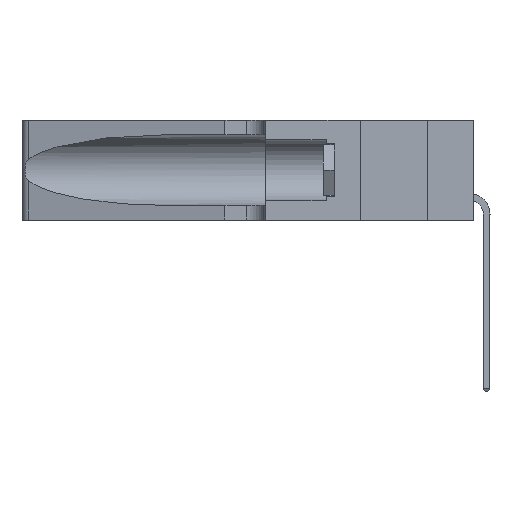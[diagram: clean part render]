
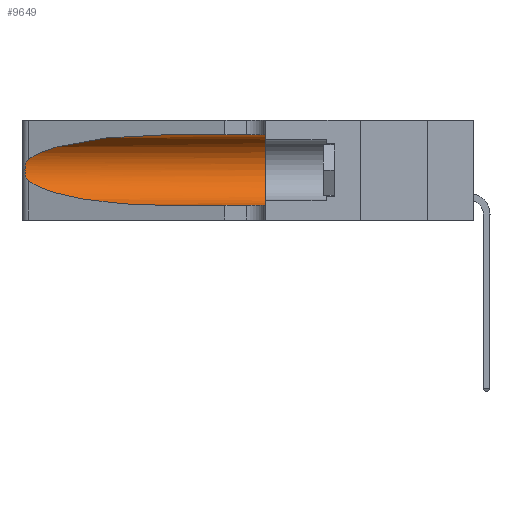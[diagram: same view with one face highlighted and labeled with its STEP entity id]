
A CAD part, left-side view. The second image highlights one B-rep face of the part: STEP entity #9649.
In plain terms, the highlighted cylindrical face has radius 3.308 mm (diameter 6.617 mm), a partial arc.
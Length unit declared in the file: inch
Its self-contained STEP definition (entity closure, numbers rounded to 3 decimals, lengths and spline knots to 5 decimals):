
#487 = CARTESIAN_POINT ( 'NONE',  ( 0.25789, 1.23486, 0.15765 ) ) ;
#1350 = VECTOR ( 'NONE', #30710, 39.37008 ) ;
#1384 = CARTESIAN_POINT ( 'NONE',  ( 0.2373, 1.15595, 0.28018 ) ) ;
#1556 = CARTESIAN_POINT ( 'NONE',  ( 0.1305, 0.72297, 0.31525 ) ) ;
#2177 = ORIENTED_EDGE ( 'NONE', *, *, #15404, .T. ) ;
#2580 = LINE ( 'NONE', #40165, #47400 ) ;
#2984 = ORIENTED_EDGE ( 'NONE', *, *, #41375, .T. ) ;
#3879 = VERTEX_POINT ( 'NONE', #7950 ) ;
#4218 = ORIENTED_EDGE ( 'NONE', *, *, #9594, .F. ) ;
#4560 = CARTESIAN_POINT ( 'NONE',  ( 0.25639, 1.23184, 0.21858 ) ) ;
#5374 =( BOUNDED_CURVE ( )  B_SPLINE_CURVE ( 3, ( #1556, #9085, #1384, #12860 ),
 .UNSPECIFIED., .F., .T. ) 
 B_SPLINE_CURVE_WITH_KNOTS ( ( 4, 4 ),
 ( 1.5708, 2.84003 ),
 .UNSPECIFIED. ) 
 CURVE ( )  GEOMETRIC_REPRESENTATION_ITEM ( )  RATIONAL_B_SPLINE_CURVE ( ( 1., 0.87, 0.87, 1. ) ) 
 REPRESENTATION_ITEM ( '' )  );
#7828 = DIRECTION ( 'NONE',  ( 0., 0., -1. ) ) ;
#7950 = CARTESIAN_POINT ( 'NONE',  ( 0.1305, 0.72297, 0.31525 ) ) ;
#9085 = CARTESIAN_POINT ( 'NONE',  ( 0.18966, 0.96281, 0.31525 ) ) ;
#9122 = ORIENTED_EDGE ( 'NONE', *, *, #40054, .T. ) ;
#9594 = EDGE_CURVE ( 'NONE', #42029, #45434, #28784, .T. ) ;
#9649 = ADVANCED_FACE ( 'NONE', ( #47097 ), #9889, .F. ) ;
#9889 = CYLINDRICAL_SURFACE ( 'NONE', #23465, 0.13025 ) ;
#11296 = CARTESIAN_POINT ( 'NONE',  ( 0.18966, 0.96281, 0.05475 ) ) ;
#11804 = CARTESIAN_POINT ( 'NONE',  ( 0.25856, 1.23593, 0.16098 ) ) ;
#11967 = CARTESIAN_POINT ( 'NONE',  ( 0.25787, 1.23484, 0.2124 ) ) ;
#12120 = CARTESIAN_POINT ( 'NONE',  ( 0.25487, 1.22718, 0.14631 ) ) ;
#12860 = CARTESIAN_POINT ( 'NONE',  ( 0.25487, 1.22718, 0.22369 ) ) ;
#14746 = CARTESIAN_POINT ( 'NONE',  ( 0.25487, 1.22718, 0.14631 ) ) ;
#15404 = EDGE_CURVE ( 'NONE', #3879, #44452, #5374, .T. ) ;
#18473 = AXIS2_PLACEMENT_3D ( 'NONE', #41687, #30249, #37850 ) ;
#18548 = CARTESIAN_POINT ( 'NONE',  ( 0.1305, 0.72297, 0.05475 ) ) ;
#19381 = CARTESIAN_POINT ( 'NONE',  ( 0.25854, 1.2359, 0.20912 ) ) ;
#19549 = CARTESIAN_POINT ( 'NONE',  ( 0.25555, 1.22994, 0.2215 ) ) ;
#19633 = CARTESIAN_POINT ( 'NONE',  ( 0.25487, 1.22718, 0.14631 ) ) ;
#22849 = CARTESIAN_POINT ( 'NONE',  ( 0.25487, 1.22718, 0.22369 ) ) ;
#23465 = AXIS2_PLACEMENT_3D ( 'NONE', #30411, #34366, #7828 ) ;
#23596 = CARTESIAN_POINT ( 'NONE',  ( 0.1305, 1.61858, 0.05475 ) ) ;
#24300 = LINE ( 'NONE', #23596, #1350 ) ;
#25050 = CARTESIAN_POINT ( 'NONE',  ( 0.1305, 0.35, 0.05475 ) ) ;
#26682 = CARTESIAN_POINT ( 'NONE',  ( 0.26017, 1.23833, 0.17102 ) ) ;
#26802 = EDGE_CURVE ( 'NONE', #3879, #42029, #2580, .T. ) ;
#28784 = CIRCLE ( 'NONE', #18473, 0.13025 ) ;
#30091 = CARTESIAN_POINT ( 'NONE',  ( 0.2373, 1.15595, 0.08982 ) ) ;
#30249 = DIRECTION ( 'NONE',  ( 0., 1., 0. ) ) ;
#30411 = CARTESIAN_POINT ( 'NONE',  ( 0.1305, 1.61858, 0.185 ) ) ;
#30710 = DIRECTION ( 'NONE',  ( 0., -1., 0. ) ) ;
#30914 = CARTESIAN_POINT ( 'NONE',  ( 0.26075, 1.23896, 0.19203 ) ) ;
#31328 = EDGE_LOOP ( 'NONE', ( #2177, #2984, #32538, #9122, #4218, #44464 ) ) ;
#32538 = ORIENTED_EDGE ( 'NONE', *, *, #48421, .T. ) ;
#33211 =( BOUNDED_CURVE ( )  B_SPLINE_CURVE ( 3, ( #14746, #30091, #11296, #18548 ),
 .UNSPECIFIED., .F., .T. ) 
 B_SPLINE_CURVE_WITH_KNOTS ( ( 4, 4 ),
 ( 3.44316, 4.71239 ),
 .UNSPECIFIED. ) 
 CURVE ( )  GEOMETRIC_REPRESENTATION_ITEM ( )  RATIONAL_B_SPLINE_CURVE ( ( 1., 0.87, 0.87, 1. ) ) 
 REPRESENTATION_ITEM ( '' )  );
#34099 = CARTESIAN_POINT ( 'NONE',  ( 0.25555, 1.22993, 0.14849 ) ) ;
#34366 = DIRECTION ( 'NONE',  ( 0., -1., 0. ) ) ;
#34716 = CARTESIAN_POINT ( 'NONE',  ( 0.26075, 1.23896, 0.178 ) ) ;
#36223 = B_SPLINE_CURVE_WITH_KNOTS ( 'NONE', 3,
 ( #22849, #19549, #4560, #11967, #19381, #45984, #30914, #34716, #26682, #11804, #487, #45384, #34099, #12120 ),
 .UNSPECIFIED., .F., .F.,
 ( 4, 2, 2, 2, 2, 2, 4 ),
 ( 0., 0.00027, 0.00053, 0.00107, 0.0016, 0.00187, 0.00214 ),
 .UNSPECIFIED. ) ;
#36700 = DIRECTION ( 'NONE',  ( 0., -1., 0. ) ) ;
#37457 = VERTEX_POINT ( 'NONE', #19633 ) ;
#37850 = DIRECTION ( 'NONE',  ( 0., 0., 1. ) ) ;
#38152 = CARTESIAN_POINT ( 'NONE',  ( 0.1305, 0.35, 0.31525 ) ) ;
#40054 = EDGE_CURVE ( 'NONE', #42758, #45434, #24300, .T. ) ;
#40165 = CARTESIAN_POINT ( 'NONE',  ( 0.1305, 1.61858, 0.31525 ) ) ;
#41375 = EDGE_CURVE ( 'NONE', #44452, #37457, #36223, .T. ) ;
#41687 = CARTESIAN_POINT ( 'NONE',  ( 0.1305, 0.35, 0.185 ) ) ;
#42029 = VERTEX_POINT ( 'NONE', #38152 ) ;
#42758 = VERTEX_POINT ( 'NONE', #46679 ) ;
#44452 = VERTEX_POINT ( 'NONE', #45171 ) ;
#44464 = ORIENTED_EDGE ( 'NONE', *, *, #26802, .F. ) ;
#45171 = CARTESIAN_POINT ( 'NONE',  ( 0.25487, 1.22718, 0.22369 ) ) ;
#45384 = CARTESIAN_POINT ( 'NONE',  ( 0.25639, 1.23186, 0.15144 ) ) ;
#45434 = VERTEX_POINT ( 'NONE', #25050 ) ;
#45984 = CARTESIAN_POINT ( 'NONE',  ( 0.26018, 1.23835, 0.19895 ) ) ;
#46679 = CARTESIAN_POINT ( 'NONE',  ( 0.1305, 0.72297, 0.05475 ) ) ;
#47097 = FACE_OUTER_BOUND ( 'NONE', #31328, .T. ) ;
#47400 = VECTOR ( 'NONE', #36700, 39.37008 ) ;
#48421 = EDGE_CURVE ( 'NONE', #37457, #42758, #33211, .T. ) ;
